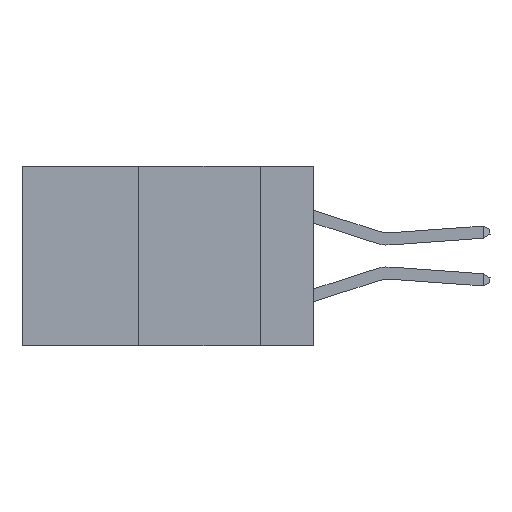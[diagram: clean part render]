
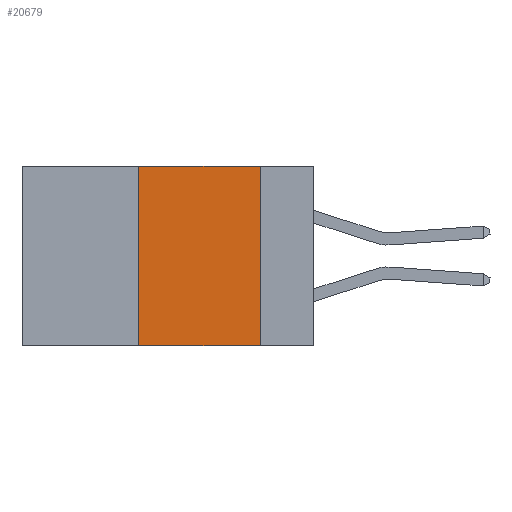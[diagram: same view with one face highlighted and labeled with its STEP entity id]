
A CAD part, left-side view. The second image highlights one B-rep face of the part: STEP entity #20679.
In plain terms, the highlighted planar face has unit normal (-1, 0, 0).
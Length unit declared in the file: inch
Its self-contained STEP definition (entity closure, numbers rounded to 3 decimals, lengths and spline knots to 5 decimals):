
#49 = CARTESIAN_POINT ( 'NONE',  ( 0., 0.6, 0. ) ) ;
#140 = DIRECTION ( 'NONE',  ( 0., 0., -1. ) ) ;
#333 = EDGE_CURVE ( 'NONE', #16066, #4079, #5960, .T. ) ;
#1274 = VECTOR ( 'NONE', #19060, 39.37008 ) ;
#1908 = EDGE_CURVE ( 'NONE', #8823, #20006, #10093, .T. ) ;
#2622 = DIRECTION ( 'NONE',  ( 0., -1., 0. ) ) ;
#4079 = VERTEX_POINT ( 'NONE', #11939 ) ;
#4979 = DIRECTION ( 'NONE',  ( 0., -1., 0. ) ) ;
#5383 = CARTESIAN_POINT ( 'NONE',  ( 0., 0.11, -0.37 ) ) ;
#5960 = LINE ( 'NONE', #12463, #1274 ) ;
#5971 = VECTOR ( 'NONE', #2622, 39.37008 ) ;
#6162 = CARTESIAN_POINT ( 'NONE',  ( 0., 0.6, -0.37 ) ) ;
#6494 = LINE ( 'NONE', #6162, #5971 ) ;
#7443 = FACE_OUTER_BOUND ( 'NONE', #19194, .T. ) ;
#8823 = VERTEX_POINT ( 'NONE', #21276 ) ;
#9228 = AXIS2_PLACEMENT_3D ( 'NONE', #49, #10492, #140 ) ;
#9566 = VECTOR ( 'NONE', #20884, 39.37008 ) ;
#10093 = LINE ( 'NONE', #16492, #9566 ) ;
#10492 = DIRECTION ( 'NONE',  ( 1., 0., 0. ) ) ;
#11939 = CARTESIAN_POINT ( 'NONE',  ( 0., 0.36, 0. ) ) ;
#12463 = CARTESIAN_POINT ( 'NONE',  ( 0., 0.36, 0. ) ) ;
#13478 = CARTESIAN_POINT ( 'NONE',  ( 0., 0.6, 0. ) ) ;
#13745 = EDGE_CURVE ( 'NONE', #16066, #20006, #6494, .T. ) ;
#14012 = ORIENTED_EDGE ( 'NONE', *, *, #13745, .T. ) ;
#14051 = ORIENTED_EDGE ( 'NONE', *, *, #333, .F. ) ;
#14282 = ORIENTED_EDGE ( 'NONE', *, *, #1908, .F. ) ;
#14298 = ORIENTED_EDGE ( 'NONE', *, *, #21812, .F. ) ;
#16066 = VERTEX_POINT ( 'NONE', #18868 ) ;
#16492 = CARTESIAN_POINT ( 'NONE',  ( 0., 0.11, 0. ) ) ;
#17293 = PLANE ( 'NONE',  #9228 ) ;
#17506 = VECTOR ( 'NONE', #4979, 39.37008 ) ;
#18537 = LINE ( 'NONE', #13478, #17506 ) ;
#18868 = CARTESIAN_POINT ( 'NONE',  ( 0., 0.36, -0.37 ) ) ;
#19060 = DIRECTION ( 'NONE',  ( 0., 0., 1. ) ) ;
#19194 = EDGE_LOOP ( 'NONE', ( #14282, #14298, #14051, #14012 ) ) ;
#20006 = VERTEX_POINT ( 'NONE', #5383 ) ;
#20679 = ADVANCED_FACE ( 'NONE', ( #7443 ), #17293, .F. ) ;
#20884 = DIRECTION ( 'NONE',  ( 0., 0., -1. ) ) ;
#21276 = CARTESIAN_POINT ( 'NONE',  ( 0., 0.11, 0. ) ) ;
#21812 = EDGE_CURVE ( 'NONE', #4079, #8823, #18537, .T. ) ;
